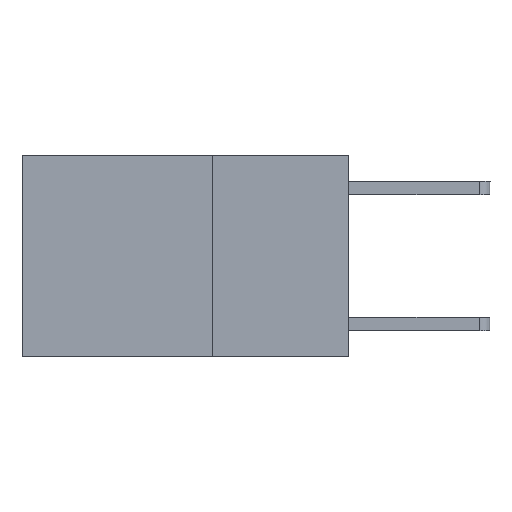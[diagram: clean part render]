
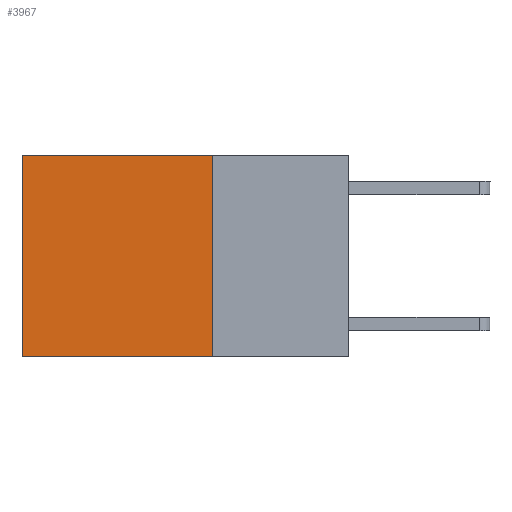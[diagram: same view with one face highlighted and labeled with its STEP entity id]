
A CAD part, left-side view. The second image highlights one B-rep face of the part: STEP entity #3967.
In plain terms, the highlighted planar face has unit normal (-1, 0, 0).
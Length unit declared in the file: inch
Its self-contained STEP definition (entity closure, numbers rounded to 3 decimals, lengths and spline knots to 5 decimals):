
#456 = EDGE_CURVE ( 'NONE', #5715, #2943, #2395, .T. ) ;
#775 = ORIENTED_EDGE ( 'NONE', *, *, #7951, .F. ) ;
#837 = DIRECTION ( 'NONE',  ( 0., 0., -1. ) ) ;
#925 = DIRECTION ( 'NONE',  ( 0., 0., -1. ) ) ;
#1029 = CARTESIAN_POINT ( 'NONE',  ( 0.2625, 0.25, 0. ) ) ;
#1285 = CARTESIAN_POINT ( 'NONE',  ( 0.2625, 0.6, -0.37 ) ) ;
#1354 = ORIENTED_EDGE ( 'NONE', *, *, #456, .T. ) ;
#1497 = VECTOR ( 'NONE', #4097, 39.37008 ) ;
#1593 = CARTESIAN_POINT ( 'NONE',  ( 0.2625, 0.25, 0. ) ) ;
#1608 = EDGE_CURVE ( 'NONE', #2943, #5591, #6645, .T. ) ;
#1702 = DIRECTION ( 'NONE',  ( 0., 1., 0. ) ) ;
#1778 = DIRECTION ( 'NONE',  ( 1., 0., 0. ) ) ;
#2395 = LINE ( 'NONE', #7401, #4987 ) ;
#2489 = EDGE_CURVE ( 'NONE', #5808, #5591, #6656, .T. ) ;
#2603 = AXIS2_PLACEMENT_3D ( 'NONE', #1029, #1778, #4278 ) ;
#2615 = VECTOR ( 'NONE', #837, 39.37008 ) ;
#2943 = VERTEX_POINT ( 'NONE', #3384 ) ;
#3329 = CARTESIAN_POINT ( 'NONE',  ( 0.2625, 0.25, 0. ) ) ;
#3384 = CARTESIAN_POINT ( 'NONE',  ( 0.2625, 0.6, 0. ) ) ;
#3451 = VECTOR ( 'NONE', #925, 39.37008 ) ;
#3516 = CARTESIAN_POINT ( 'NONE',  ( 0.2625, 0.25, -0.37 ) ) ;
#3530 = CARTESIAN_POINT ( 'NONE',  ( 0.2625, 0.25, -0.37 ) ) ;
#3967 = ADVANCED_FACE ( 'NONE', ( #5528 ), #4811, .F. ) ;
#4097 = DIRECTION ( 'NONE',  ( 0., 1., 0. ) ) ;
#4259 = LINE ( 'NONE', #1593, #3451 ) ;
#4278 = DIRECTION ( 'NONE',  ( 0., 0., -1. ) ) ;
#4811 = PLANE ( 'NONE',  #2603 ) ;
#4987 = VECTOR ( 'NONE', #1702, 39.37008 ) ;
#5104 = EDGE_LOOP ( 'NONE', ( #7122, #5115, #775, #1354 ) ) ;
#5115 = ORIENTED_EDGE ( 'NONE', *, *, #2489, .F. ) ;
#5528 = FACE_OUTER_BOUND ( 'NONE', #5104, .T. ) ;
#5591 = VERTEX_POINT ( 'NONE', #1285 ) ;
#5715 = VERTEX_POINT ( 'NONE', #3329 ) ;
#5808 = VERTEX_POINT ( 'NONE', #3530 ) ;
#6510 = CARTESIAN_POINT ( 'NONE',  ( 0.2625, 0.6, 0. ) ) ;
#6645 = LINE ( 'NONE', #6510, #2615 ) ;
#6656 = LINE ( 'NONE', #3516, #1497 ) ;
#7122 = ORIENTED_EDGE ( 'NONE', *, *, #1608, .T. ) ;
#7401 = CARTESIAN_POINT ( 'NONE',  ( 0.2625, 0.25, 0. ) ) ;
#7951 = EDGE_CURVE ( 'NONE', #5715, #5808, #4259, .T. ) ;
